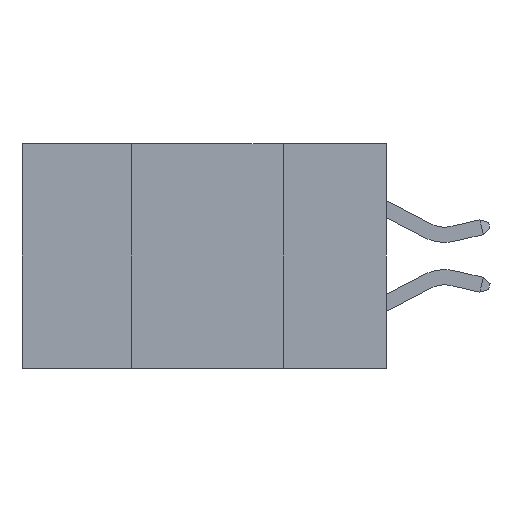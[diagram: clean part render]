
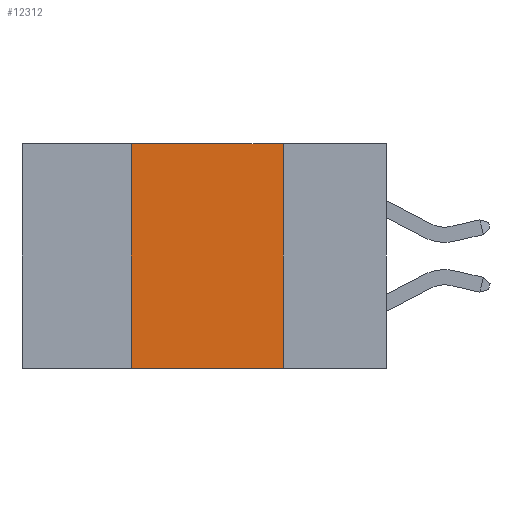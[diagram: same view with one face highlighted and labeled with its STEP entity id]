
A CAD part, left-side view. The second image highlights one B-rep face of the part: STEP entity #12312.
In plain terms, the highlighted planar face has unit normal (-1, 0, 0).
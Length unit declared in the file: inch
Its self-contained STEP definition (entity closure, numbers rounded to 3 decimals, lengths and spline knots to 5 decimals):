
#430 = EDGE_CURVE ( 'NONE', #7237, #4784, #1891, .T. ) ;
#671 = ORIENTED_EDGE ( 'NONE', *, *, #5001, .T. ) ;
#1246 = DIRECTION ( 'NONE',  ( 1., 0., 0. ) ) ;
#1692 = DIRECTION ( 'NONE',  ( 0., -1., 0. ) ) ;
#1891 = LINE ( 'NONE', #23132, #15929 ) ;
#2185 = CARTESIAN_POINT ( 'NONE',  ( 0., 0.42, 0. ) ) ;
#3029 = CARTESIAN_POINT ( 'NONE',  ( 0., 0.17, -0.37 ) ) ;
#3195 = CARTESIAN_POINT ( 'NONE',  ( 0., 0.17, 0. ) ) ;
#4524 = EDGE_CURVE ( 'NONE', #4784, #12654, #8262, .T. ) ;
#4784 = VERTEX_POINT ( 'NONE', #2185 ) ;
#5001 = EDGE_CURVE ( 'NONE', #7237, #18497, #20277, .T. ) ;
#5315 = FACE_OUTER_BOUND ( 'NONE', #22098, .T. ) ;
#7237 = VERTEX_POINT ( 'NONE', #10223 ) ;
#8262 = LINE ( 'NONE', #21316, #16951 ) ;
#8432 = DIRECTION ( 'NONE',  ( 0., 0., -1. ) ) ;
#9864 = DIRECTION ( 'NONE',  ( 0., -1., 0. ) ) ;
#10223 = CARTESIAN_POINT ( 'NONE',  ( 0., 0.42, -0.37 ) ) ;
#11598 = ORIENTED_EDGE ( 'NONE', *, *, #4524, .F. ) ;
#11808 = LINE ( 'NONE', #18266, #14316 ) ;
#11973 = CARTESIAN_POINT ( 'NONE',  ( 0., 0.6, 0. ) ) ;
#12312 = ADVANCED_FACE ( 'NONE', ( #5315 ), #17594, .F. ) ;
#12354 = ORIENTED_EDGE ( 'NONE', *, *, #430, .F. ) ;
#12654 = VERTEX_POINT ( 'NONE', #3195 ) ;
#14316 = VECTOR ( 'NONE', #21877, 39.37008 ) ;
#14359 = DIRECTION ( 'NONE',  ( 0., 0., 1. ) ) ;
#15929 = VECTOR ( 'NONE', #14359, 39.37008 ) ;
#16245 = ORIENTED_EDGE ( 'NONE', *, *, #17021, .F. ) ;
#16636 = VECTOR ( 'NONE', #9864, 39.37008 ) ;
#16951 = VECTOR ( 'NONE', #1692, 39.37008 ) ;
#17021 = EDGE_CURVE ( 'NONE', #12654, #18497, #11808, .T. ) ;
#17594 = PLANE ( 'NONE',  #20504 ) ;
#18266 = CARTESIAN_POINT ( 'NONE',  ( 0., 0.17, 0. ) ) ;
#18497 = VERTEX_POINT ( 'NONE', #3029 ) ;
#20277 = LINE ( 'NONE', #20513, #16636 ) ;
#20504 = AXIS2_PLACEMENT_3D ( 'NONE', #11973, #1246, #8432 ) ;
#20513 = CARTESIAN_POINT ( 'NONE',  ( 0., 0.6, -0.37 ) ) ;
#21316 = CARTESIAN_POINT ( 'NONE',  ( 0., 0.6, 0. ) ) ;
#21877 = DIRECTION ( 'NONE',  ( 0., 0., -1. ) ) ;
#22098 = EDGE_LOOP ( 'NONE', ( #16245, #11598, #12354, #671 ) ) ;
#23132 = CARTESIAN_POINT ( 'NONE',  ( 0., 0.42, 0. ) ) ;
